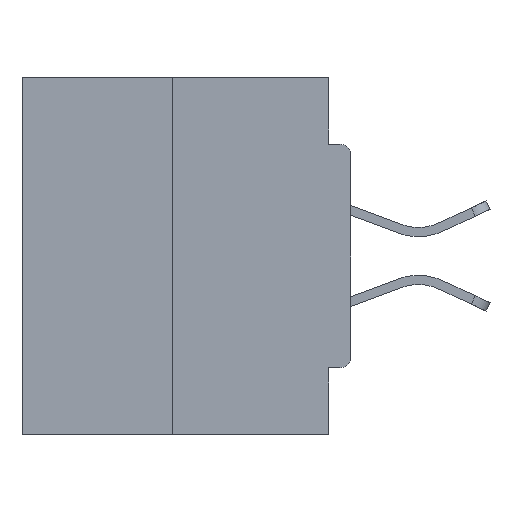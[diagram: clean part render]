
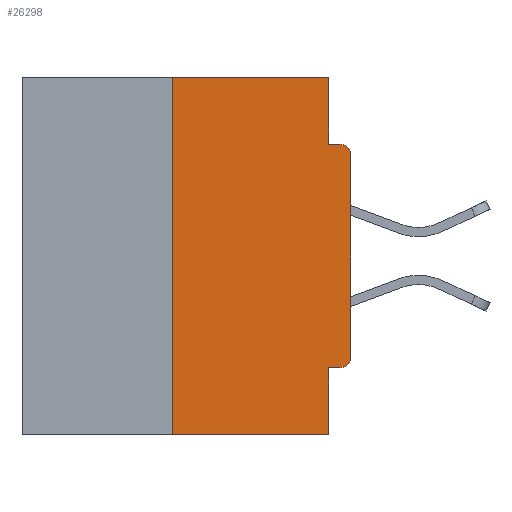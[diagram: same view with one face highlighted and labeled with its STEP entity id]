
A CAD part, left-side view. The second image highlights one B-rep face of the part: STEP entity #26298.
In plain terms, the highlighted planar face has unit normal (-1, 0, 0).
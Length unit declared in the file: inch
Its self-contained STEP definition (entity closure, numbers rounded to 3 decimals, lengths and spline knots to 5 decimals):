
#960 = DIRECTION ( 'NONE',  ( 0., 0., -1. ) ) ;
#1621 = CARTESIAN_POINT ( 'NONE',  ( 0., 0., -0.0935 ) ) ;
#1890 = CARTESIAN_POINT ( 'NONE',  ( 0., 0.031, -0.0935 ) ) ;
#2221 = LINE ( 'NONE', #33782, #4539 ) ;
#2589 = DIRECTION ( 'NONE',  ( 0., 1., 0. ) ) ;
#3339 = EDGE_CURVE ( 'NONE', #28592, #33184, #4320, .T. ) ;
#3421 = LINE ( 'NONE', #1621, #25105 ) ;
#3895 = DIRECTION ( 'NONE',  ( 0., -1., 0. ) ) ;
#3941 = VERTEX_POINT ( 'NONE', #16514 ) ;
#4124 = DIRECTION ( 'NONE',  ( 0., 0., -1. ) ) ;
#4320 = LINE ( 'NONE', #12454, #30185 ) ;
#4431 = CARTESIAN_POINT ( 'NONE',  ( 0., 0.46, 0. ) ) ;
#4539 = VECTOR ( 'NONE', #3895, 39.37008 ) ;
#4713 = ORIENTED_EDGE ( 'NONE', *, *, #6618, .F. ) ;
#4747 = DIRECTION ( 'NONE',  ( 0., 0., 1. ) ) ;
#4873 = VERTEX_POINT ( 'NONE', #35613 ) ;
#5099 = DIRECTION ( 'NONE',  ( -1., 0., 0. ) ) ;
#5945 = VECTOR ( 'NONE', #16600, 39.37008 ) ;
#6618 = EDGE_CURVE ( 'NONE', #7134, #27811, #10398, .T. ) ;
#7134 = VERTEX_POINT ( 'NONE', #27762 ) ;
#7546 = CARTESIAN_POINT ( 'NONE',  ( 0., 0.46, 0. ) ) ;
#8061 = VECTOR ( 'NONE', #18185, 39.37008 ) ;
#8539 = CARTESIAN_POINT ( 'NONE',  ( 0., 0.031, 0. ) ) ;
#9155 = LINE ( 'NONE', #37801, #10548 ) ;
#10357 = LINE ( 'NONE', #29878, #8061 ) ;
#10398 = LINE ( 'NONE', #16267, #27914 ) ;
#10423 = EDGE_CURVE ( 'NONE', #27811, #10894, #22055, .T. ) ;
#10502 = EDGE_CURVE ( 'NONE', #35425, #3941, #37748, .T. ) ;
#10548 = VECTOR ( 'NONE', #2589, 39.37008 ) ;
#10894 = VERTEX_POINT ( 'NONE', #8539 ) ;
#11509 = CARTESIAN_POINT ( 'NONE',  ( 0., 0.031, -0.5 ) ) ;
#11636 = AXIS2_PLACEMENT_3D ( 'NONE', #25355, #13766, #25240 ) ;
#12454 = CARTESIAN_POINT ( 'NONE',  ( 0., 0.031, -0.5 ) ) ;
#12688 = EDGE_CURVE ( 'NONE', #7134, #33184, #2221, .T. ) ;
#13766 = DIRECTION ( 'NONE',  ( -1., 0., 0. ) ) ;
#14136 = DIRECTION ( 'NONE',  ( 0., 0., -1. ) ) ;
#16085 = FACE_OUTER_BOUND ( 'NONE', #33676, .T. ) ;
#16267 = CARTESIAN_POINT ( 'NONE',  ( 0., 0.25, 0. ) ) ;
#16514 = CARTESIAN_POINT ( 'NONE',  ( 0., 0., -0.3915 ) ) ;
#16600 = DIRECTION ( 'NONE',  ( 0., -1., 0. ) ) ;
#18185 = DIRECTION ( 'NONE',  ( 0., 0., 1. ) ) ;
#18283 = PLANE ( 'NONE',  #18487 ) ;
#18487 = AXIS2_PLACEMENT_3D ( 'NONE', #4431, #19296, #33811 ) ;
#19034 = ORIENTED_EDGE ( 'NONE', *, *, #10423, .F. ) ;
#19116 = CARTESIAN_POINT ( 'NONE',  ( 0., 0.031, 0. ) ) ;
#19296 = DIRECTION ( 'NONE',  ( 1., 0., 0. ) ) ;
#19448 = DIRECTION ( 'NONE',  ( 0., -1., 0. ) ) ;
#20875 = ORIENTED_EDGE ( 'NONE', *, *, #29247, .T. ) ;
#21038 = ORIENTED_EDGE ( 'NONE', *, *, #10502, .T. ) ;
#22055 = LINE ( 'NONE', #7546, #5945 ) ;
#23233 = EDGE_CURVE ( 'NONE', #10894, #30706, #23324, .T. ) ;
#23324 = LINE ( 'NONE', #19116, #24238 ) ;
#23497 = ORIENTED_EDGE ( 'NONE', *, *, #37258, .F. ) ;
#24238 = VECTOR ( 'NONE', #4124, 39.37008 ) ;
#25105 = VECTOR ( 'NONE', #19448, 39.37008 ) ;
#25240 = DIRECTION ( 'NONE',  ( 0., 0., -1. ) ) ;
#25355 = CARTESIAN_POINT ( 'NONE',  ( 0., 0.015, -0.1085 ) ) ;
#25874 = CARTESIAN_POINT ( 'NONE',  ( 0., 0.015, -0.3915 ) ) ;
#26298 = ADVANCED_FACE ( 'NONE', ( #16085 ), #18283, .F. ) ;
#26408 = EDGE_CURVE ( 'NONE', #35425, #28592, #9155, .T. ) ;
#27084 = AXIS2_PLACEMENT_3D ( 'NONE', #25874, #5099, #14136 ) ;
#27762 = CARTESIAN_POINT ( 'NONE',  ( 0., 0.25, -0.5 ) ) ;
#27811 = VERTEX_POINT ( 'NONE', #30794 ) ;
#27914 = VECTOR ( 'NONE', #4747, 39.37008 ) ;
#28592 = VERTEX_POINT ( 'NONE', #36999 ) ;
#29247 = EDGE_CURVE ( 'NONE', #29935, #4873, #32874, .T. ) ;
#29373 = ORIENTED_EDGE ( 'NONE', *, *, #12688, .T. ) ;
#29483 = CARTESIAN_POINT ( 'NONE',  ( 0., 0.015, -0.4065 ) ) ;
#29878 = CARTESIAN_POINT ( 'NONE',  ( 0., 0., 0. ) ) ;
#29935 = VERTEX_POINT ( 'NONE', #31108 ) ;
#30185 = VECTOR ( 'NONE', #960, 39.37008 ) ;
#30379 = ORIENTED_EDGE ( 'NONE', *, *, #3339, .F. ) ;
#30706 = VERTEX_POINT ( 'NONE', #1890 ) ;
#30794 = CARTESIAN_POINT ( 'NONE',  ( 0., 0.25, 0. ) ) ;
#31029 = ORIENTED_EDGE ( 'NONE', *, *, #23233, .F. ) ;
#31108 = CARTESIAN_POINT ( 'NONE',  ( 0., 0., -0.1085 ) ) ;
#31349 = ORIENTED_EDGE ( 'NONE', *, *, #26408, .F. ) ;
#32874 = CIRCLE ( 'NONE', #11636, 0.015 ) ;
#33184 = VERTEX_POINT ( 'NONE', #11509 ) ;
#33676 = EDGE_LOOP ( 'NONE', ( #19034, #4713, #29373, #30379, #31349, #21038, #35976, #20875, #23497, #31029 ) ) ;
#33782 = CARTESIAN_POINT ( 'NONE',  ( 0., 0.46, -0.5 ) ) ;
#33811 = DIRECTION ( 'NONE',  ( 0., 0., -1. ) ) ;
#35425 = VERTEX_POINT ( 'NONE', #29483 ) ;
#35613 = CARTESIAN_POINT ( 'NONE',  ( 0., 0.015, -0.0935 ) ) ;
#35976 = ORIENTED_EDGE ( 'NONE', *, *, #36934, .T. ) ;
#36934 = EDGE_CURVE ( 'NONE', #3941, #29935, #10357, .T. ) ;
#36999 = CARTESIAN_POINT ( 'NONE',  ( 0., 0.031, -0.4065 ) ) ;
#37258 = EDGE_CURVE ( 'NONE', #30706, #4873, #3421, .T. ) ;
#37748 = CIRCLE ( 'NONE', #27084, 0.015 ) ;
#37801 = CARTESIAN_POINT ( 'NONE',  ( 0., 0., -0.4065 ) ) ;
